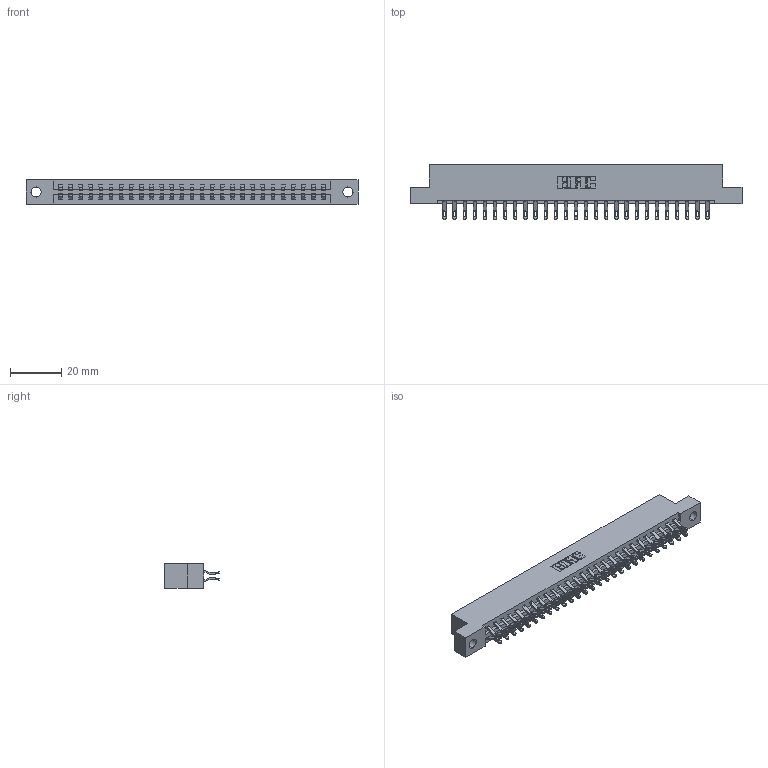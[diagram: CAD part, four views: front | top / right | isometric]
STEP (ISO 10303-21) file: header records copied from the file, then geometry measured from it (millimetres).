
FILE_DESCRIPTION (( 'STEP AP203' ), '1' );
FILE_NAME ('387-054-555-204.STEP', '2019-10-19T05:25:11', ( '' ), ( '' ), 'SwSTEP 2.0', 'SolidWorks 2016', '' );
FILE_SCHEMA (( 'CONFIG_CONTROL_DESIGN' ));
Length unit declared in the file: inch
Products named in the file (3): 337 Part_Flush Mounting Lugs - 0.156 Dia-TH; 387-054-555-204; 345-292-001_555 Tail
Assembly tree (55 placements, depth 2):
  387-054-555-204
    337 Part_Flush Mounting Lugs - 0.156 Dia-TH
    345-292-001_555 Tail  x54
Bounding box: 130 x 21.47 x 9.4 mm (x, y, z)
Volume: 13569.2 mm3; surface area: 15582 mm2
Topology: 55 solids, 55 shells, 3354 faces, 10517 edges, 7010 vertices
Faces by surface type: plane 2014, cylinder 1340
Entity records: 23203 total; most frequent: CARTESIAN_POINT 3956, ORIENTED_EDGE 3862, DIRECTION 3363, EDGE_CURVE 1931, VECTOR 1783, LINE 1783, VERTEX_POINT 1286, AXIS2_PLACEMENT_3D 790
